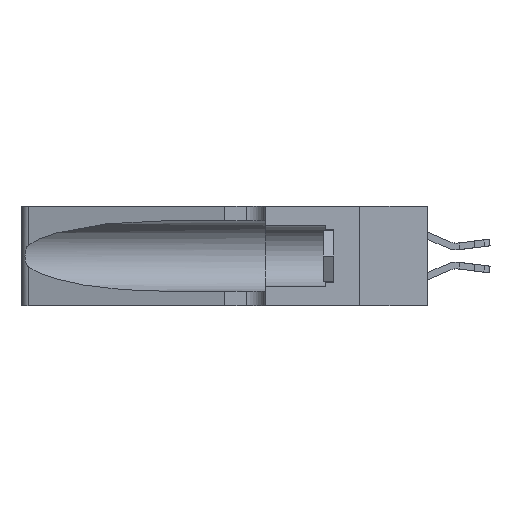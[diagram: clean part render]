
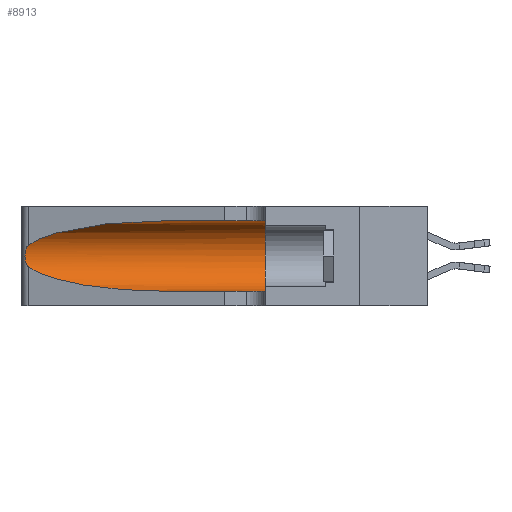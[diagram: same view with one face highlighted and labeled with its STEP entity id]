
A CAD part, left-side view. The second image highlights one B-rep face of the part: STEP entity #8913.
In plain terms, the highlighted cylindrical face has radius 3.308 mm (diameter 6.617 mm), a partial arc.
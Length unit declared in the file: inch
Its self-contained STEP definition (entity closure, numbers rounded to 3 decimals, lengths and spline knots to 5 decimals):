
#245 = VERTEX_POINT ( 'NONE', #9016 ) ;
#722 = EDGE_CURVE ( 'NONE', #6336, #25551, #23633, .T. ) ;
#1765 = CARTESIAN_POINT ( 'NONE',  ( 0.26075, 1.23896, 0.178 ) ) ;
#1777 = EDGE_CURVE ( 'NONE', #6336, #6115, #22374, .T. ) ;
#1803 = DIRECTION ( 'NONE',  ( 0., 0., 1. ) ) ;
#1852 = CARTESIAN_POINT ( 'NONE',  ( 0.25487, 1.22718, 0.22369 ) ) ;
#2133 = CARTESIAN_POINT ( 'NONE',  ( 0.25787, 1.23484, 0.2124 ) ) ;
#2535 = CYLINDRICAL_SURFACE ( 'NONE', #21135, 0.13025 ) ;
#2727 = ORIENTED_EDGE ( 'NONE', *, *, #722, .F. ) ;
#2873 = DIRECTION ( 'NONE',  ( 0., -1., 0. ) ) ;
#3202 = CARTESIAN_POINT ( 'NONE',  ( 0.1305, 0.72297, 0.31525 ) ) ;
#3306 = VECTOR ( 'NONE', #21393, 39.37008 ) ;
#3937 = CARTESIAN_POINT ( 'NONE',  ( 0.25856, 1.23593, 0.16098 ) ) ;
#3972 = CARTESIAN_POINT ( 'NONE',  ( 0.2373, 1.15595, 0.28018 ) ) ;
#4287 = CARTESIAN_POINT ( 'NONE',  ( 0.25854, 1.2359, 0.20912 ) ) ;
#5881 = FACE_OUTER_BOUND ( 'NONE', #23369, .T. ) ;
#5983 = ORIENTED_EDGE ( 'NONE', *, *, #16212, .T. ) ;
#6115 = VERTEX_POINT ( 'NONE', #15502 ) ;
#6327 = CARTESIAN_POINT ( 'NONE',  ( 0.26017, 1.23833, 0.17102 ) ) ;
#6336 = VERTEX_POINT ( 'NONE', #15216 ) ;
#7299 = CARTESIAN_POINT ( 'NONE',  ( 0.18966, 0.96281, 0.05475 ) ) ;
#7738 = ORIENTED_EDGE ( 'NONE', *, *, #1777, .T. ) ;
#7761 = CARTESIAN_POINT ( 'NONE',  ( 0.1305, 1.61858, 0.185 ) ) ;
#8026 = B_SPLINE_CURVE_WITH_KNOTS ( 'NONE', 3,
 ( #1852, #23142, #16910, #2133, #4287, #8306, #10369, #1765, #6327, #3937, #14798, #25251, #23395, #16999 ),
 .UNSPECIFIED., .F., .F.,
 ( 4, 2, 2, 2, 2, 2, 4 ),
 ( 0., 0.00027, 0.00053, 0.00107, 0.0016, 0.00187, 0.00214 ),
 .UNSPECIFIED. ) ;
#8250 = CARTESIAN_POINT ( 'NONE',  ( 0.1305, 0.35, 0.31525 ) ) ;
#8306 = CARTESIAN_POINT ( 'NONE',  ( 0.26018, 1.23835, 0.19895 ) ) ;
#8357 = DIRECTION ( 'NONE',  ( 0., 1., 0. ) ) ;
#8913 = ADVANCED_FACE ( 'NONE', ( #5881 ), #2535, .F. ) ;
#9016 = CARTESIAN_POINT ( 'NONE',  ( 0.1305, 0.72297, 0.05475 ) ) ;
#10369 = CARTESIAN_POINT ( 'NONE',  ( 0.26075, 1.23896, 0.19203 ) ) ;
#10636 = ORIENTED_EDGE ( 'NONE', *, *, #11182, .T. ) ;
#11182 = EDGE_CURVE ( 'NONE', #24258, #245, #24904, .T. ) ;
#11386 = DIRECTION ( 'NONE',  ( 0., 0., -1. ) ) ;
#13209 = LINE ( 'NONE', #14005, #27032 ) ;
#14005 = CARTESIAN_POINT ( 'NONE',  ( 0.1305, 1.61858, 0.05475 ) ) ;
#14782 = CIRCLE ( 'NONE', #17222, 0.13025 ) ;
#14798 = CARTESIAN_POINT ( 'NONE',  ( 0.25789, 1.23486, 0.15765 ) ) ;
#14963 = EDGE_CURVE ( 'NONE', #25551, #25689, #14782, .T. ) ;
#15216 = CARTESIAN_POINT ( 'NONE',  ( 0.1305, 0.72297, 0.31525 ) ) ;
#15502 = CARTESIAN_POINT ( 'NONE',  ( 0.25487, 1.22718, 0.22369 ) ) ;
#15893 = ORIENTED_EDGE ( 'NONE', *, *, #14963, .F. ) ;
#16015 = CARTESIAN_POINT ( 'NONE',  ( 0.2373, 1.15595, 0.08982 ) ) ;
#16212 = EDGE_CURVE ( 'NONE', #6115, #24258, #8026, .T. ) ;
#16910 = CARTESIAN_POINT ( 'NONE',  ( 0.25639, 1.23184, 0.21858 ) ) ;
#16999 = CARTESIAN_POINT ( 'NONE',  ( 0.25487, 1.22718, 0.14631 ) ) ;
#17222 = AXIS2_PLACEMENT_3D ( 'NONE', #27372, #8357, #1803 ) ;
#17874 = ORIENTED_EDGE ( 'NONE', *, *, #21869, .T. ) ;
#18224 = CARTESIAN_POINT ( 'NONE',  ( 0.1305, 0.72297, 0.05475 ) ) ;
#18611 = CARTESIAN_POINT ( 'NONE',  ( 0.1305, 1.61858, 0.31525 ) ) ;
#20284 = CARTESIAN_POINT ( 'NONE',  ( 0.18966, 0.96281, 0.31525 ) ) ;
#21135 = AXIS2_PLACEMENT_3D ( 'NONE', #7761, #23394, #11386 ) ;
#21350 = CARTESIAN_POINT ( 'NONE',  ( 0.25487, 1.22718, 0.22369 ) ) ;
#21393 = DIRECTION ( 'NONE',  ( 0., -1., 0. ) ) ;
#21869 = EDGE_CURVE ( 'NONE', #245, #25689, #13209, .T. ) ;
#22374 =( BOUNDED_CURVE ( )  B_SPLINE_CURVE ( 3, ( #3202, #20284, #3972, #21350 ),
 .UNSPECIFIED., .F., .F. ) 
 B_SPLINE_CURVE_WITH_KNOTS ( ( 4, 4 ),
 ( 1.5708, 2.84003 ),
 .UNSPECIFIED. ) 
 CURVE ( )  GEOMETRIC_REPRESENTATION_ITEM ( )  RATIONAL_B_SPLINE_CURVE ( ( 1., 0.87, 0.87, 1. ) ) 
 REPRESENTATION_ITEM ( '' )  );
#23142 = CARTESIAN_POINT ( 'NONE',  ( 0.25555, 1.22994, 0.2215 ) ) ;
#23369 = EDGE_LOOP ( 'NONE', ( #7738, #5983, #10636, #17874, #15893, #2727 ) ) ;
#23394 = DIRECTION ( 'NONE',  ( 0., -1., 0. ) ) ;
#23395 = CARTESIAN_POINT ( 'NONE',  ( 0.25555, 1.22993, 0.14849 ) ) ;
#23425 = CARTESIAN_POINT ( 'NONE',  ( 0.1305, 0.35, 0.05475 ) ) ;
#23633 = LINE ( 'NONE', #18611, #3306 ) ;
#24258 = VERTEX_POINT ( 'NONE', #25148 ) ;
#24691 = CARTESIAN_POINT ( 'NONE',  ( 0.25487, 1.22718, 0.14631 ) ) ;
#24904 =( BOUNDED_CURVE ( )  B_SPLINE_CURVE ( 3, ( #24691, #16015, #7299, #18224 ),
 .UNSPECIFIED., .F., .F. ) 
 B_SPLINE_CURVE_WITH_KNOTS ( ( 4, 4 ),
 ( 3.44316, 4.71239 ),
 .UNSPECIFIED. ) 
 CURVE ( )  GEOMETRIC_REPRESENTATION_ITEM ( )  RATIONAL_B_SPLINE_CURVE ( ( 1., 0.87, 0.87, 1. ) ) 
 REPRESENTATION_ITEM ( '' )  );
#25148 = CARTESIAN_POINT ( 'NONE',  ( 0.25487, 1.22718, 0.14631 ) ) ;
#25251 = CARTESIAN_POINT ( 'NONE',  ( 0.25639, 1.23186, 0.15144 ) ) ;
#25551 = VERTEX_POINT ( 'NONE', #8250 ) ;
#25689 = VERTEX_POINT ( 'NONE', #23425 ) ;
#27032 = VECTOR ( 'NONE', #2873, 39.37008 ) ;
#27372 = CARTESIAN_POINT ( 'NONE',  ( 0.1305, 0.35, 0.185 ) ) ;
